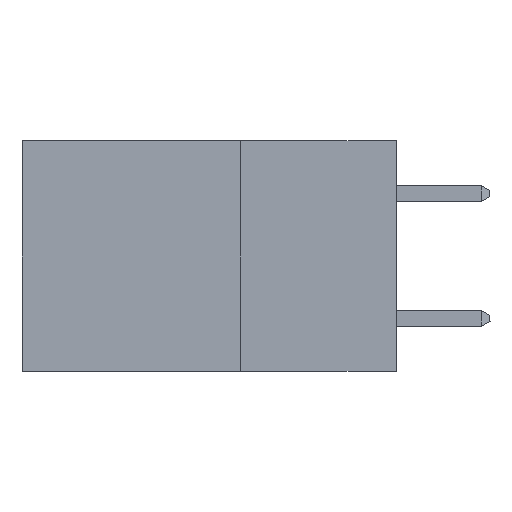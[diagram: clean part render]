
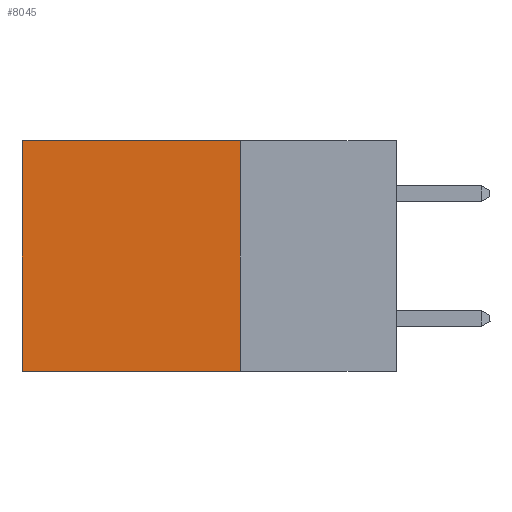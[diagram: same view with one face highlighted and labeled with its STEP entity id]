
A CAD part, left-side view. The second image highlights one B-rep face of the part: STEP entity #8045.
In plain terms, the highlighted planar face has unit normal (-1, 0, 0).
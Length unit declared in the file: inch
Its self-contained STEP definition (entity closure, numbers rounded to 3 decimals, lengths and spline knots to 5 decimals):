
#1838 = ORIENTED_EDGE ( 'NONE', *, *, #18976, .F. ) ;
#1891 = ORIENTED_EDGE ( 'NONE', *, *, #9334, .F. ) ;
#2626 = VECTOR ( 'NONE', #5156, 39.37008 ) ;
#4229 = VERTEX_POINT ( 'NONE', #22877 ) ;
#5156 = DIRECTION ( 'NONE',  ( 0., 0., -1. ) ) ;
#8045 = ADVANCED_FACE ( 'NONE', ( #11393 ), #18494, .F. ) ;
#8303 = VERTEX_POINT ( 'NONE', #15399 ) ;
#9334 = EDGE_CURVE ( 'NONE', #4229, #8303, #13288, .T. ) ;
#10887 = DIRECTION ( 'NONE',  ( 0., 0., -1. ) ) ;
#11393 = FACE_OUTER_BOUND ( 'NONE', #21964, .T. ) ;
#12367 = CARTESIAN_POINT ( 'NONE',  ( 0.2615, 0.25, 0. ) ) ;
#12546 = CARTESIAN_POINT ( 'NONE',  ( 0.2615, 0.6, 0. ) ) ;
#12777 = VERTEX_POINT ( 'NONE', #20283 ) ;
#12820 = CARTESIAN_POINT ( 'NONE',  ( 0.2615, 0.25, -0.37 ) ) ;
#13238 = DIRECTION ( 'NONE',  ( 0., 0., -1. ) ) ;
#13288 = LINE ( 'NONE', #20760, #17743 ) ;
#13522 = LINE ( 'NONE', #12367, #17965 ) ;
#14298 = DIRECTION ( 'NONE',  ( 0., 1., 0. ) ) ;
#15281 = VERTEX_POINT ( 'NONE', #12546 ) ;
#15399 = CARTESIAN_POINT ( 'NONE',  ( 0.2615, 0.25, -0.37 ) ) ;
#16640 = CARTESIAN_POINT ( 'NONE',  ( 0.2615, 0.6, -0.37 ) ) ;
#17308 = LINE ( 'NONE', #16640, #2626 ) ;
#17743 = VECTOR ( 'NONE', #13238, 39.37008 ) ;
#17965 = VECTOR ( 'NONE', #14298, 39.37008 ) ;
#18040 = LINE ( 'NONE', #12820, #22459 ) ;
#18494 = PLANE ( 'NONE',  #20589 ) ;
#18555 = DIRECTION ( 'NONE',  ( 0., 1., 0. ) ) ;
#18976 = EDGE_CURVE ( 'NONE', #8303, #12777, #18040, .T. ) ;
#19998 = ORIENTED_EDGE ( 'NONE', *, *, #22587, .T. ) ;
#20283 = CARTESIAN_POINT ( 'NONE',  ( 0.2615, 0.6, -0.37 ) ) ;
#20589 = AXIS2_PLACEMENT_3D ( 'NONE', #22175, #22269, #10887 ) ;
#20760 = CARTESIAN_POINT ( 'NONE',  ( 0.2615, 0.25, -0.37 ) ) ;
#21964 = EDGE_LOOP ( 'NONE', ( #24044, #1838, #1891, #19998 ) ) ;
#22175 = CARTESIAN_POINT ( 'NONE',  ( 0.2615, 0.25, -0.37 ) ) ;
#22269 = DIRECTION ( 'NONE',  ( 1., 0., 0. ) ) ;
#22459 = VECTOR ( 'NONE', #18555, 39.37008 ) ;
#22587 = EDGE_CURVE ( 'NONE', #4229, #15281, #13522, .T. ) ;
#22877 = CARTESIAN_POINT ( 'NONE',  ( 0.2615, 0.25, 0. ) ) ;
#24001 = EDGE_CURVE ( 'NONE', #15281, #12777, #17308, .T. ) ;
#24044 = ORIENTED_EDGE ( 'NONE', *, *, #24001, .T. ) ;
